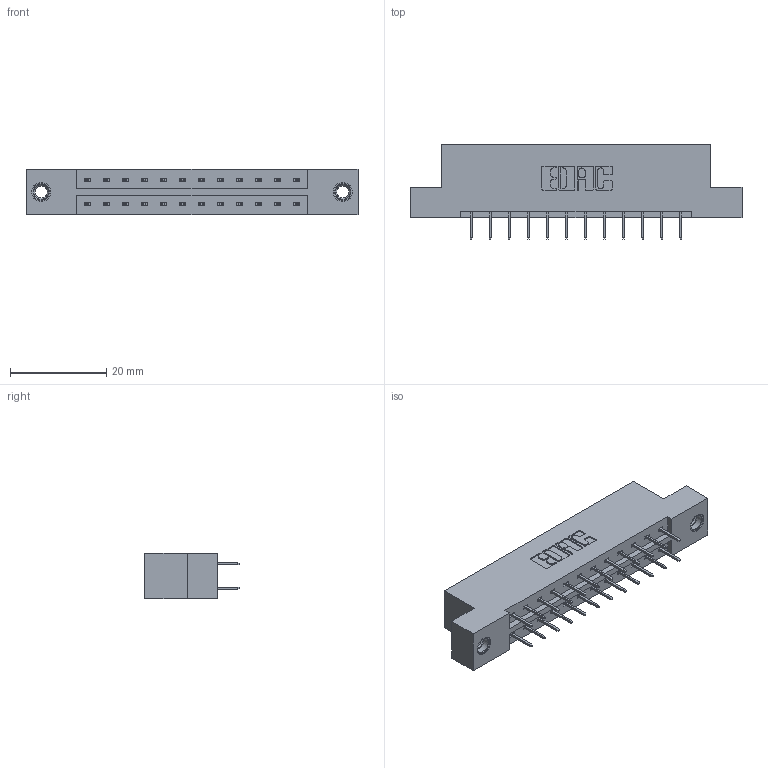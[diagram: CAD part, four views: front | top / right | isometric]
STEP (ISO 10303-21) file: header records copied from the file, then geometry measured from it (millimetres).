
FILE_DESCRIPTION (( 'STEP AP203' ), '1' );
FILE_NAME ('833-024-524-207.STEP', '2020-06-01T20:57:03', ( '' ), ( '' ), 'SwSTEP 2.0', 'SolidWorks 2020', '' );
FILE_SCHEMA (( 'CONFIG_CONTROL_DESIGN' ));
Length unit declared in the file: inch
Products named in the file (4): 833-024-524-207; 833 Part_Flush - .156 Dia - TI; 345-250-001_345-250-005-103; 345-292-001_345-293-124
Assembly tree (27 placements, depth 2):
  833-024-524-207
    833 Part_Flush - .156 Dia - TI
    345-292-001_345-293-124  x24
    345-250-001_345-250-005-103  x2
Bounding box: 69.09 x 19.69 x 9.4 mm (x, y, z)
Volume: 6723.1 mm3; surface area: 7551.1 mm2
Topology: 27 solids, 27 shells, 1518 faces, 4263 edges, 2738 vertices
Faces by surface type: plane 1110, cylinder 392, cone 12, torus 4
Entity records: 12860 total; most frequent: CARTESIAN_POINT 2149, ORIENTED_EDGE 2078, DIRECTION 1921, EDGE_CURVE 1039, LINE 895, VECTOR 895, VERTEX_POINT 684, AXIS2_PLACEMENT_3D 513
